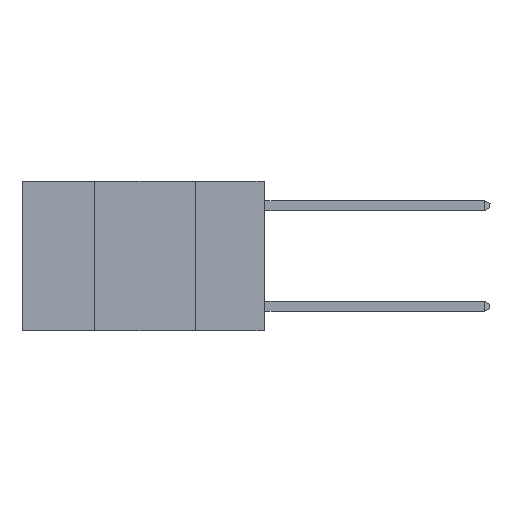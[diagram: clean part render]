
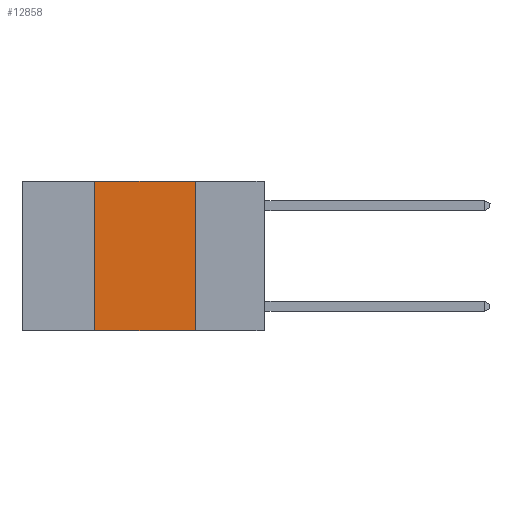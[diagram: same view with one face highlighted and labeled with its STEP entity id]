
A CAD part, left-side view. The second image highlights one B-rep face of the part: STEP entity #12858.
In plain terms, the highlighted planar face has unit normal (-1, 0, 0).
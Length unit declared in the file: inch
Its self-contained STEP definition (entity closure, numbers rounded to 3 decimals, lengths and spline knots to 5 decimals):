
#1241 = LINE ( 'NONE', #6683, #14492 ) ;
#2706 = CARTESIAN_POINT ( 'NONE',  ( 0., 0.17, -0.37 ) ) ;
#5147 = PLANE ( 'NONE',  #6204 ) ;
#5523 = FACE_OUTER_BOUND ( 'NONE', #9372, .T. ) ;
#5729 = CARTESIAN_POINT ( 'NONE',  ( 0., 0.6, 0. ) ) ;
#6204 = AXIS2_PLACEMENT_3D ( 'NONE', #20369, #8777, #13062 ) ;
#6657 = CARTESIAN_POINT ( 'NONE',  ( 0., 0.42, -0.37 ) ) ;
#6683 = CARTESIAN_POINT ( 'NONE',  ( 0., 0.42, 0. ) ) ;
#8777 = DIRECTION ( 'NONE',  ( 1., 0., 0. ) ) ;
#8822 = ORIENTED_EDGE ( 'NONE', *, *, #16230, .F. ) ;
#8867 = CARTESIAN_POINT ( 'NONE',  ( 0., 0.17, 0. ) ) ;
#9137 = LINE ( 'NONE', #14955, #17590 ) ;
#9372 = EDGE_LOOP ( 'NONE', ( #21918, #8822, #23561, #11676 ) ) ;
#9693 = VERTEX_POINT ( 'NONE', #8867 ) ;
#10928 = DIRECTION ( 'NONE',  ( 0., 0., 1. ) ) ;
#11279 = EDGE_CURVE ( 'NONE', #12704, #16001, #9137, .T. ) ;
#11676 = ORIENTED_EDGE ( 'NONE', *, *, #11279, .T. ) ;
#12704 = VERTEX_POINT ( 'NONE', #6657 ) ;
#12858 = ADVANCED_FACE ( 'NONE', ( #5523 ), #5147, .F. ) ;
#13062 = DIRECTION ( 'NONE',  ( 0., 0., -1. ) ) ;
#14492 = VECTOR ( 'NONE', #10928, 39.37008 ) ;
#14955 = CARTESIAN_POINT ( 'NONE',  ( 0., 0.6, -0.37 ) ) ;
#16001 = VERTEX_POINT ( 'NONE', #2706 ) ;
#16230 = EDGE_CURVE ( 'NONE', #19556, #9693, #21343, .T. ) ;
#17564 = CARTESIAN_POINT ( 'NONE',  ( 0., 0.17, 0. ) ) ;
#17590 = VECTOR ( 'NONE', #18583, 39.37008 ) ;
#18583 = DIRECTION ( 'NONE',  ( 0., -1., 0. ) ) ;
#19429 = CARTESIAN_POINT ( 'NONE',  ( 0., 0.42, 0. ) ) ;
#19438 = LINE ( 'NONE', #17564, #23317 ) ;
#19556 = VERTEX_POINT ( 'NONE', #19429 ) ;
#20369 = CARTESIAN_POINT ( 'NONE',  ( 0., 0.6, 0. ) ) ;
#21218 = DIRECTION ( 'NONE',  ( 0., -1., 0. ) ) ;
#21343 = LINE ( 'NONE', #5729, #24757 ) ;
#21529 = EDGE_CURVE ( 'NONE', #9693, #16001, #19438, .T. ) ;
#21918 = ORIENTED_EDGE ( 'NONE', *, *, #21529, .F. ) ;
#23317 = VECTOR ( 'NONE', #23384, 39.37008 ) ;
#23384 = DIRECTION ( 'NONE',  ( 0., 0., -1. ) ) ;
#23561 = ORIENTED_EDGE ( 'NONE', *, *, #23918, .F. ) ;
#23918 = EDGE_CURVE ( 'NONE', #12704, #19556, #1241, .T. ) ;
#24757 = VECTOR ( 'NONE', #21218, 39.37008 ) ;
